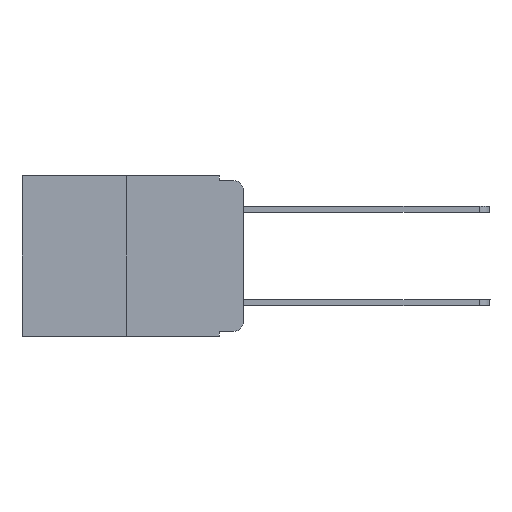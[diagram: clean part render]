
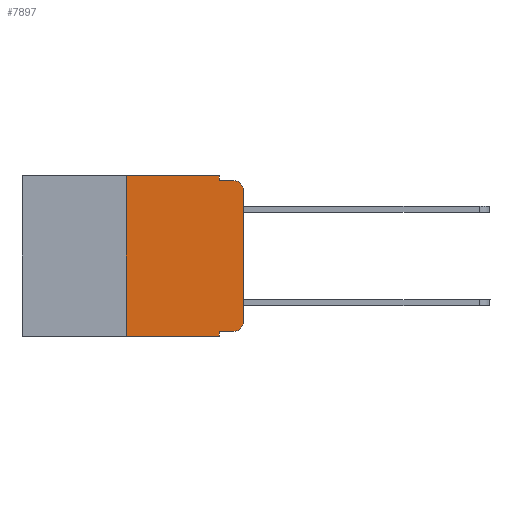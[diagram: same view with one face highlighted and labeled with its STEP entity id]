
A CAD part, left-side view. The second image highlights one B-rep face of the part: STEP entity #7897.
In plain terms, the highlighted planar face has unit normal (-1, 0, 0).
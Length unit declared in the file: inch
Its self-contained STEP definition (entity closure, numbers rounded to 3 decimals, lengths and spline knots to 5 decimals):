
#60 = EDGE_CURVE ( 'NONE', #3169, #6979, #10090, .T. ) ;
#209 = DIRECTION ( 'NONE',  ( -1., 0., 0. ) ) ;
#249 = VECTOR ( 'NONE', #6085, 39.37008 ) ;
#391 = CARTESIAN_POINT ( 'NONE',  ( 0., 0.051, -0.343 ) ) ;
#407 = CARTESIAN_POINT ( 'NONE',  ( 0., 0., 0. ) ) ;
#445 = CARTESIAN_POINT ( 'NONE',  ( 0., 0.25, 0. ) ) ;
#480 = FACE_OUTER_BOUND ( 'NONE', #5165, .T. ) ;
#531 = CARTESIAN_POINT ( 'NONE',  ( 0., 0.473, -0.343 ) ) ;
#578 = CARTESIAN_POINT ( 'NONE',  ( 0., 0.051, -0.333 ) ) ;
#642 = EDGE_CURVE ( 'NONE', #3769, #6577, #10339, .T. ) ;
#650 = DIRECTION ( 'NONE',  ( 0., 0., -1. ) ) ;
#683 = CARTESIAN_POINT ( 'NONE',  ( 0., 0.25, -0.343 ) ) ;
#699 = ORIENTED_EDGE ( 'NONE', *, *, #1497, .T. ) ;
#1007 = LINE ( 'NONE', #578, #9389 ) ;
#1225 = ORIENTED_EDGE ( 'NONE', *, *, #60, .F. ) ;
#1284 = CARTESIAN_POINT ( 'NONE',  ( 0., 0.02, -0.01 ) ) ;
#1497 = EDGE_CURVE ( 'NONE', #4367, #7561, #9226, .T. ) ;
#1598 = ORIENTED_EDGE ( 'NONE', *, *, #4070, .T. ) ;
#1788 = DIRECTION ( 'NONE',  ( 0., -1., 0. ) ) ;
#2072 = AXIS2_PLACEMENT_3D ( 'NONE', #4303, #7653, #9972 ) ;
#2187 = AXIS2_PLACEMENT_3D ( 'NONE', #7234, #7193, #8004 ) ;
#2194 = DIRECTION ( 'NONE',  ( 0., -1., 0. ) ) ;
#2385 = VERTEX_POINT ( 'NONE', #1284 ) ;
#2401 = VECTOR ( 'NONE', #7309, 39.37008 ) ;
#2590 = DIRECTION ( 'NONE',  ( 0., 0., -1. ) ) ;
#2743 = VECTOR ( 'NONE', #4516, 39.37008 ) ;
#2930 = VERTEX_POINT ( 'NONE', #391 ) ;
#2939 = EDGE_CURVE ( 'NONE', #6979, #2385, #5102, .T. ) ;
#3045 = VERTEX_POINT ( 'NONE', #9381 ) ;
#3088 = LINE ( 'NONE', #531, #4712 ) ;
#3169 = VERTEX_POINT ( 'NONE', #7946 ) ;
#3509 = CARTESIAN_POINT ( 'NONE',  ( 0., 0.051, -0.01 ) ) ;
#3729 = EDGE_CURVE ( 'NONE', #3769, #2930, #3088, .T. ) ;
#3769 = VERTEX_POINT ( 'NONE', #683 ) ;
#3940 = LINE ( 'NONE', #407, #249 ) ;
#4070 = EDGE_CURVE ( 'NONE', #7561, #7175, #3940, .T. ) ;
#4303 = CARTESIAN_POINT ( 'NONE',  ( 0., 0.02, -0.313 ) ) ;
#4367 = VERTEX_POINT ( 'NONE', #4899 ) ;
#4516 = DIRECTION ( 'NONE',  ( 0., 0., 1. ) ) ;
#4554 = CARTESIAN_POINT ( 'NONE',  ( 0., 0.051, -0.01 ) ) ;
#4636 = CARTESIAN_POINT ( 'NONE',  ( 0., 0.051, 0. ) ) ;
#4712 = VECTOR ( 'NONE', #7172, 39.37008 ) ;
#4854 = ORIENTED_EDGE ( 'NONE', *, *, #2939, .F. ) ;
#4899 = CARTESIAN_POINT ( 'NONE',  ( 0., 0.02, -0.333 ) ) ;
#5102 = LINE ( 'NONE', #3509, #5996 ) ;
#5165 = EDGE_LOOP ( 'NONE', ( #1598, #6939, #4854, #1225, #5972, #6335, #5943, #7797, #5998, #699 ) ) ;
#5602 = CARTESIAN_POINT ( 'NONE',  ( 0., 0.25, 0. ) ) ;
#5943 = ORIENTED_EDGE ( 'NONE', *, *, #3729, .T. ) ;
#5972 = ORIENTED_EDGE ( 'NONE', *, *, #7283, .F. ) ;
#5996 = VECTOR ( 'NONE', #10094, 39.37008 ) ;
#5998 = ORIENTED_EDGE ( 'NONE', *, *, #6357, .T. ) ;
#6085 = DIRECTION ( 'NONE',  ( 0., 0., 1. ) ) ;
#6335 = ORIENTED_EDGE ( 'NONE', *, *, #642, .F. ) ;
#6357 = EDGE_CURVE ( 'NONE', #3045, #4367, #1007, .T. ) ;
#6415 = EDGE_CURVE ( 'NONE', #3045, #2930, #10231, .T. ) ;
#6577 = VERTEX_POINT ( 'NONE', #5602 ) ;
#6881 = CARTESIAN_POINT ( 'NONE',  ( 0., 0., -0.313 ) ) ;
#6939 = ORIENTED_EDGE ( 'NONE', *, *, #7442, .T. ) ;
#6979 = VERTEX_POINT ( 'NONE', #4554 ) ;
#7172 = DIRECTION ( 'NONE',  ( 0., -1., 0. ) ) ;
#7175 = VERTEX_POINT ( 'NONE', #10401 ) ;
#7193 = DIRECTION ( 'NONE',  ( 1., 0., 0. ) ) ;
#7234 = CARTESIAN_POINT ( 'NONE',  ( 0., 0.473, 0. ) ) ;
#7283 = EDGE_CURVE ( 'NONE', #6577, #3169, #10355, .T. ) ;
#7309 = DIRECTION ( 'NONE',  ( 0., 0., -1. ) ) ;
#7328 = VECTOR ( 'NONE', #1788, 39.37008 ) ;
#7442 = EDGE_CURVE ( 'NONE', #7175, #2385, #9476, .T. ) ;
#7561 = VERTEX_POINT ( 'NONE', #6881 ) ;
#7653 = DIRECTION ( 'NONE',  ( -1., 0., 0. ) ) ;
#7670 = AXIS2_PLACEMENT_3D ( 'NONE', #8264, #209, #2590 ) ;
#7797 = ORIENTED_EDGE ( 'NONE', *, *, #6415, .F. ) ;
#7897 = ADVANCED_FACE ( 'NONE', ( #480 ), #8812, .F. ) ;
#7946 = CARTESIAN_POINT ( 'NONE',  ( 0., 0.051, 0. ) ) ;
#8004 = DIRECTION ( 'NONE',  ( 0., 0., -1. ) ) ;
#8264 = CARTESIAN_POINT ( 'NONE',  ( 0., 0.02, -0.03 ) ) ;
#8812 = PLANE ( 'NONE',  #2187 ) ;
#8944 = CARTESIAN_POINT ( 'NONE',  ( 0., 0.473, 0. ) ) ;
#9226 = CIRCLE ( 'NONE', #2072, 0.02 ) ;
#9381 = CARTESIAN_POINT ( 'NONE',  ( 0., 0.051, -0.333 ) ) ;
#9389 = VECTOR ( 'NONE', #2194, 39.37008 ) ;
#9476 = CIRCLE ( 'NONE', #7670, 0.02 ) ;
#9630 = VECTOR ( 'NONE', #650, 39.37008 ) ;
#9772 = CARTESIAN_POINT ( 'NONE',  ( 0., 0.051, 0. ) ) ;
#9972 = DIRECTION ( 'NONE',  ( 0., 0., -1. ) ) ;
#10090 = LINE ( 'NONE', #9772, #2401 ) ;
#10094 = DIRECTION ( 'NONE',  ( 0., -1., 0. ) ) ;
#10231 = LINE ( 'NONE', #4636, #9630 ) ;
#10339 = LINE ( 'NONE', #445, #2743 ) ;
#10355 = LINE ( 'NONE', #8944, #7328 ) ;
#10401 = CARTESIAN_POINT ( 'NONE',  ( 0., 0., -0.03 ) ) ;
